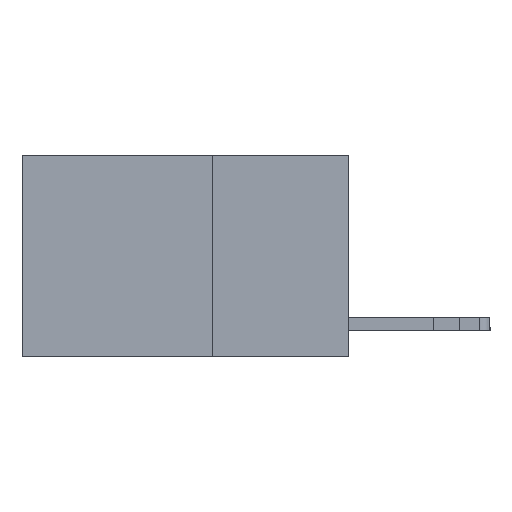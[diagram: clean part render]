
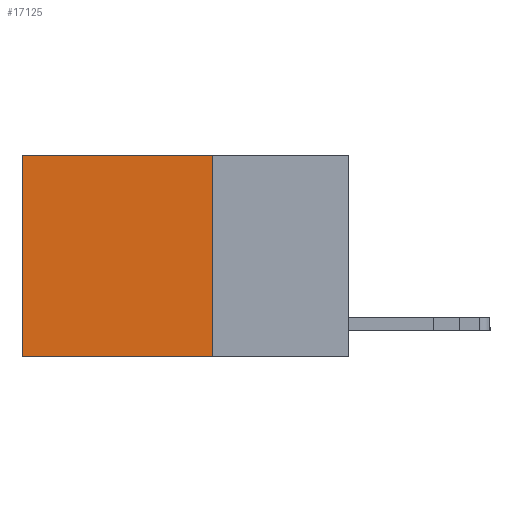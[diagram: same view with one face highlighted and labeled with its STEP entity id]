
A CAD part, left-side view. The second image highlights one B-rep face of the part: STEP entity #17125.
In plain terms, the highlighted planar face has unit normal (-1, 0, 0).
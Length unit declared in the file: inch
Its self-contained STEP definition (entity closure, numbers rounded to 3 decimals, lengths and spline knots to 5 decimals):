
#502 = AXIS2_PLACEMENT_3D ( 'NONE', #7065, #1162, #17764 ) ;
#612 = CARTESIAN_POINT ( 'NONE',  ( 0.2625, 0.25, -0.37 ) ) ;
#785 = CARTESIAN_POINT ( 'NONE',  ( 0.2625, 0.6, 0. ) ) ;
#868 = CARTESIAN_POINT ( 'NONE',  ( 0.2625, 0.25, 0. ) ) ;
#1162 = DIRECTION ( 'NONE',  ( 1., 0., 0. ) ) ;
#1377 = LINE ( 'NONE', #5661, #3099 ) ;
#2144 = VECTOR ( 'NONE', #17216, 39.37008 ) ;
#2196 = LINE ( 'NONE', #8273, #11538 ) ;
#2861 = ORIENTED_EDGE ( 'NONE', *, *, #5676, .F. ) ;
#3099 = VECTOR ( 'NONE', #15955, 39.37008 ) ;
#4398 = ORIENTED_EDGE ( 'NONE', *, *, #6428, .F. ) ;
#5129 = LINE ( 'NONE', #785, #2144 ) ;
#5661 = CARTESIAN_POINT ( 'NONE',  ( 0.2625, 0.25, 0. ) ) ;
#5676 = EDGE_CURVE ( 'NONE', #17242, #13431, #18650, .T. ) ;
#6428 = EDGE_CURVE ( 'NONE', #13431, #10102, #2196, .T. ) ;
#6889 = DIRECTION ( 'NONE',  ( 0., 0., -1. ) ) ;
#7065 = CARTESIAN_POINT ( 'NONE',  ( 0.2625, 0.25, 0. ) ) ;
#7458 = ORIENTED_EDGE ( 'NONE', *, *, #13486, .T. ) ;
#8192 = DIRECTION ( 'NONE',  ( 0., 1., 0. ) ) ;
#8273 = CARTESIAN_POINT ( 'NONE',  ( 0.2625, 0.25, -0.37 ) ) ;
#9291 = EDGE_LOOP ( 'NONE', ( #7458, #4398, #2861, #17126 ) ) ;
#10102 = VERTEX_POINT ( 'NONE', #17748 ) ;
#11001 = VERTEX_POINT ( 'NONE', #17059 ) ;
#11206 = VECTOR ( 'NONE', #6889, 39.37008 ) ;
#11538 = VECTOR ( 'NONE', #8192, 39.37008 ) ;
#12260 = CARTESIAN_POINT ( 'NONE',  ( 0.2625, 0.25, 0. ) ) ;
#13431 = VERTEX_POINT ( 'NONE', #612 ) ;
#13486 = EDGE_CURVE ( 'NONE', #11001, #10102, #5129, .T. ) ;
#13611 = EDGE_CURVE ( 'NONE', #17242, #11001, #1377, .T. ) ;
#15955 = DIRECTION ( 'NONE',  ( 0., 1., 0. ) ) ;
#16295 = FACE_OUTER_BOUND ( 'NONE', #9291, .T. ) ;
#17059 = CARTESIAN_POINT ( 'NONE',  ( 0.2625, 0.6, 0. ) ) ;
#17125 = ADVANCED_FACE ( 'NONE', ( #16295 ), #17474, .F. ) ;
#17126 = ORIENTED_EDGE ( 'NONE', *, *, #13611, .T. ) ;
#17216 = DIRECTION ( 'NONE',  ( 0., 0., -1. ) ) ;
#17242 = VERTEX_POINT ( 'NONE', #12260 ) ;
#17474 = PLANE ( 'NONE',  #502 ) ;
#17748 = CARTESIAN_POINT ( 'NONE',  ( 0.2625, 0.6, -0.37 ) ) ;
#17764 = DIRECTION ( 'NONE',  ( 0., 0., -1. ) ) ;
#18650 = LINE ( 'NONE', #868, #11206 ) ;
